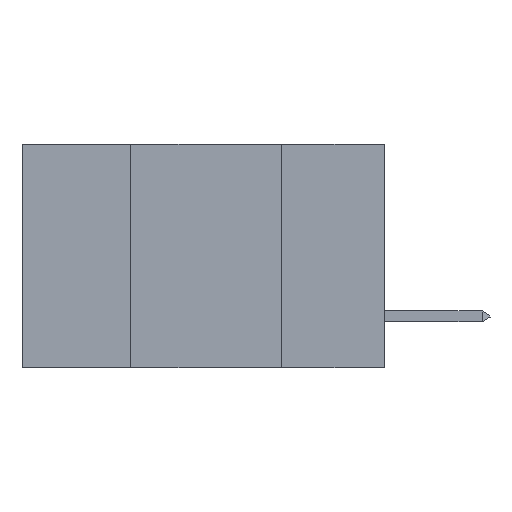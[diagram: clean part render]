
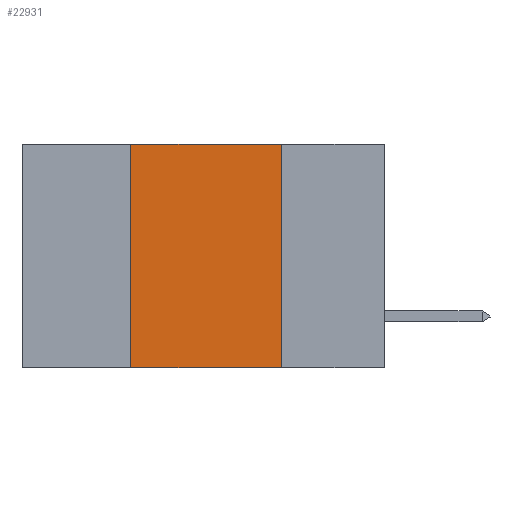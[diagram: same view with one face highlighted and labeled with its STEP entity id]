
A CAD part, left-side view. The second image highlights one B-rep face of the part: STEP entity #22931.
In plain terms, the highlighted planar face has unit normal (-1, 0, 0).
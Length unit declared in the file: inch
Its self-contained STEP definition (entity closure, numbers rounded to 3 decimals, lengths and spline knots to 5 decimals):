
#949 = CARTESIAN_POINT ( 'NONE',  ( 0., 0.6, 0. ) ) ;
#4165 = LINE ( 'NONE', #6777, #23673 ) ;
#4182 = PLANE ( 'NONE',  #9046 ) ;
#4762 = CARTESIAN_POINT ( 'NONE',  ( 0., 0.17, -0.37 ) ) ;
#6635 = DIRECTION ( 'NONE',  ( 0., 0., 1. ) ) ;
#6679 = ORIENTED_EDGE ( 'NONE', *, *, #42262, .F. ) ;
#6777 = CARTESIAN_POINT ( 'NONE',  ( 0., 0.42, 0. ) ) ;
#8598 = LINE ( 'NONE', #30051, #21833 ) ;
#9046 = AXIS2_PLACEMENT_3D ( 'NONE', #949, #13971, #20580 ) ;
#11023 = VECTOR ( 'NONE', #39829, 39.37008 ) ;
#11531 = CARTESIAN_POINT ( 'NONE',  ( 0., 0.42, 0. ) ) ;
#12911 = VERTEX_POINT ( 'NONE', #4762 ) ;
#13971 = DIRECTION ( 'NONE',  ( 1., 0., 0. ) ) ;
#14320 = CARTESIAN_POINT ( 'NONE',  ( 0., 0.42, -0.37 ) ) ;
#15488 = ORIENTED_EDGE ( 'NONE', *, *, #16545, .F. ) ;
#16545 = EDGE_CURVE ( 'NONE', #39728, #35687, #8598, .T. ) ;
#18266 = VERTEX_POINT ( 'NONE', #14320 ) ;
#19105 = DIRECTION ( 'NONE',  ( 0., 0., -1. ) ) ;
#19908 = CARTESIAN_POINT ( 'NONE',  ( 0., 0.6, -0.37 ) ) ;
#20580 = DIRECTION ( 'NONE',  ( 0., 0., -1. ) ) ;
#21037 = EDGE_CURVE ( 'NONE', #18266, #12911, #36781, .T. ) ;
#21833 = VECTOR ( 'NONE', #33124, 39.37008 ) ;
#22427 = VECTOR ( 'NONE', #19105, 39.37008 ) ;
#22931 = ADVANCED_FACE ( 'NONE', ( #25654 ), #4182, .F. ) ;
#23673 = VECTOR ( 'NONE', #6635, 39.37008 ) ;
#25654 = FACE_OUTER_BOUND ( 'NONE', #43505, .T. ) ;
#27539 = ORIENTED_EDGE ( 'NONE', *, *, #39318, .F. ) ;
#29228 = CARTESIAN_POINT ( 'NONE',  ( 0., 0.17, 0. ) ) ;
#30051 = CARTESIAN_POINT ( 'NONE',  ( 0., 0.6, 0. ) ) ;
#33124 = DIRECTION ( 'NONE',  ( 0., -1., 0. ) ) ;
#33397 = LINE ( 'NONE', #29228, #22427 ) ;
#34637 = ORIENTED_EDGE ( 'NONE', *, *, #21037, .T. ) ;
#35687 = VERTEX_POINT ( 'NONE', #40098 ) ;
#36781 = LINE ( 'NONE', #19908, #11023 ) ;
#39318 = EDGE_CURVE ( 'NONE', #35687, #12911, #33397, .T. ) ;
#39728 = VERTEX_POINT ( 'NONE', #11531 ) ;
#39829 = DIRECTION ( 'NONE',  ( 0., -1., 0. ) ) ;
#40098 = CARTESIAN_POINT ( 'NONE',  ( 0., 0.17, 0. ) ) ;
#42262 = EDGE_CURVE ( 'NONE', #18266, #39728, #4165, .T. ) ;
#43505 = EDGE_LOOP ( 'NONE', ( #27539, #15488, #6679, #34637 ) ) ;
